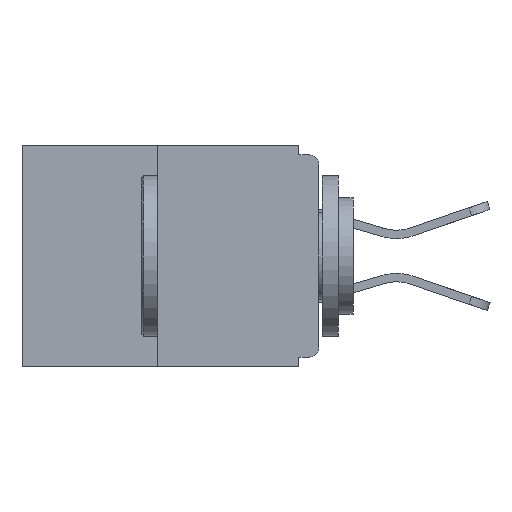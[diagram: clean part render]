
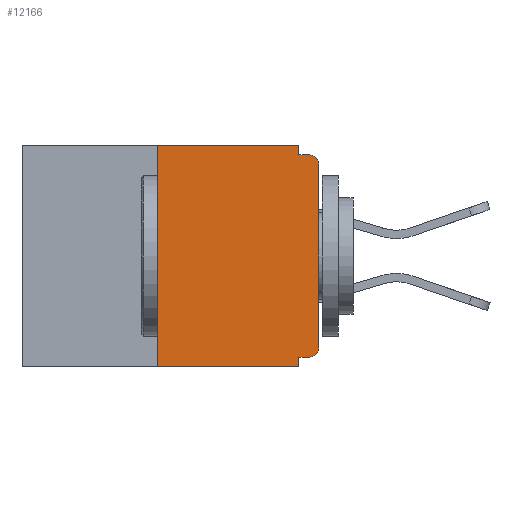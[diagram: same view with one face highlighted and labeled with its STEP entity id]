
A CAD part, left-side view. The second image highlights one B-rep face of the part: STEP entity #12166.
In plain terms, the highlighted planar face has unit normal (-1, 0, 0).
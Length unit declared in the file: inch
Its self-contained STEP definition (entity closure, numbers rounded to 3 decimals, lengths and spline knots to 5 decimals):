
#251 = EDGE_CURVE ( 'NONE', #6789, #2099, #13063, .T. ) ;
#456 = VERTEX_POINT ( 'NONE', #16855 ) ;
#589 = CARTESIAN_POINT ( 'NONE',  ( 0., 0.031, -0.015 ) ) ;
#648 = VECTOR ( 'NONE', #12299, 39.37008 ) ;
#949 = CARTESIAN_POINT ( 'NONE',  ( 0., 0.46, -0.343 ) ) ;
#1015 = DIRECTION ( 'NONE',  ( 0., -1., 0. ) ) ;
#1018 = ORIENTED_EDGE ( 'NONE', *, *, #12444, .F. ) ;
#1489 = ORIENTED_EDGE ( 'NONE', *, *, #14130, .F. ) ;
#1553 = ORIENTED_EDGE ( 'NONE', *, *, #16051, .T. ) ;
#2029 = VECTOR ( 'NONE', #5635, 39.37008 ) ;
#2099 = VERTEX_POINT ( 'NONE', #11036 ) ;
#2513 = CARTESIAN_POINT ( 'NONE',  ( 0., 0.031, -0.328 ) ) ;
#2523 = VECTOR ( 'NONE', #14605, 39.37008 ) ;
#3146 = VERTEX_POINT ( 'NONE', #15047 ) ;
#3176 = VECTOR ( 'NONE', #1015, 39.37008 ) ;
#3281 = EDGE_LOOP ( 'NONE', ( #15553, #9394, #1553, #1018, #1489, #11393, #9842, #7065, #14509, #13046 ) ) ;
#4202 = CARTESIAN_POINT ( 'NONE',  ( 0., 0.031, 0. ) ) ;
#5271 = CARTESIAN_POINT ( 'NONE',  ( 0., 0.031, 0. ) ) ;
#5534 = CARTESIAN_POINT ( 'NONE',  ( 0., 0.25, -0.343 ) ) ;
#5581 = DIRECTION ( 'NONE',  ( 0., -1., 0. ) ) ;
#5635 = DIRECTION ( 'NONE',  ( 0., 0., -1. ) ) ;
#5746 = VECTOR ( 'NONE', #5581, 39.37008 ) ;
#5886 = LINE ( 'NONE', #949, #3176 ) ;
#6510 = AXIS2_PLACEMENT_3D ( 'NONE', #8123, #16675, #8061 ) ;
#6789 = VERTEX_POINT ( 'NONE', #589 ) ;
#6872 = AXIS2_PLACEMENT_3D ( 'NONE', #17075, #10003, #14261 ) ;
#7065 = ORIENTED_EDGE ( 'NONE', *, *, #11221, .T. ) ;
#7157 = LINE ( 'NONE', #15218, #18271 ) ;
#7294 = CIRCLE ( 'NONE', #6872, 0.015 ) ;
#7665 = VERTEX_POINT ( 'NONE', #11870 ) ;
#7759 = EDGE_CURVE ( 'NONE', #15912, #6789, #17613, .T. ) ;
#8061 = DIRECTION ( 'NONE',  ( 0., 0., -1. ) ) ;
#8123 = CARTESIAN_POINT ( 'NONE',  ( 0., 0.46, 0. ) ) ;
#8216 = EDGE_CURVE ( 'NONE', #7665, #18246, #7157, .T. ) ;
#9111 = CIRCLE ( 'NONE', #14252, 0.015 ) ;
#9394 = ORIENTED_EDGE ( 'NONE', *, *, #18094, .F. ) ;
#9842 = ORIENTED_EDGE ( 'NONE', *, *, #8216, .T. ) ;
#10003 = DIRECTION ( 'NONE',  ( -1., 0., 0. ) ) ;
#10218 = VECTOR ( 'NONE', #15487, 39.37008 ) ;
#10864 = CARTESIAN_POINT ( 'NONE',  ( 0., 0., -0.03 ) ) ;
#11036 = CARTESIAN_POINT ( 'NONE',  ( 0., 0.015, -0.015 ) ) ;
#11221 = EDGE_CURVE ( 'NONE', #18246, #2099, #7294, .T. ) ;
#11393 = ORIENTED_EDGE ( 'NONE', *, *, #17899, .T. ) ;
#11527 = LINE ( 'NONE', #12703, #5746 ) ;
#11870 = CARTESIAN_POINT ( 'NONE',  ( 0., 0., -0.313 ) ) ;
#12135 = FACE_OUTER_BOUND ( 'NONE', #3281, .T. ) ;
#12145 = VECTOR ( 'NONE', #15330, 39.37008 ) ;
#12166 = ADVANCED_FACE ( 'NONE', ( #12135 ), #16099, .F. ) ;
#12299 = DIRECTION ( 'NONE',  ( 0., 1., 0. ) ) ;
#12444 = EDGE_CURVE ( 'NONE', #13809, #456, #14600, .T. ) ;
#12703 = CARTESIAN_POINT ( 'NONE',  ( 0., 0.46, 0. ) ) ;
#12765 = VERTEX_POINT ( 'NONE', #5534 ) ;
#13046 = ORIENTED_EDGE ( 'NONE', *, *, #7759, .F. ) ;
#13063 = LINE ( 'NONE', #18193, #12145 ) ;
#13226 = CARTESIAN_POINT ( 'NONE',  ( 0., 0.015, -0.313 ) ) ;
#13809 = VERTEX_POINT ( 'NONE', #2513 ) ;
#13900 = EDGE_CURVE ( 'NONE', #14069, #15912, #11527, .T. ) ;
#14011 = CARTESIAN_POINT ( 'NONE',  ( 0., 0.25, 0. ) ) ;
#14069 = VERTEX_POINT ( 'NONE', #17996 ) ;
#14130 = EDGE_CURVE ( 'NONE', #3146, #13809, #14848, .T. ) ;
#14252 = AXIS2_PLACEMENT_3D ( 'NONE', #13226, #14586, #14643 ) ;
#14261 = DIRECTION ( 'NONE',  ( 0., 0., -1. ) ) ;
#14509 = ORIENTED_EDGE ( 'NONE', *, *, #251, .F. ) ;
#14586 = DIRECTION ( 'NONE',  ( -1., 0., 0. ) ) ;
#14600 = LINE ( 'NONE', #17318, #2523 ) ;
#14605 = DIRECTION ( 'NONE',  ( 0., 0., -1. ) ) ;
#14643 = DIRECTION ( 'NONE',  ( 0., 0., -1. ) ) ;
#14848 = LINE ( 'NONE', #15141, #648 ) ;
#15047 = CARTESIAN_POINT ( 'NONE',  ( 0., 0.015, -0.328 ) ) ;
#15141 = CARTESIAN_POINT ( 'NONE',  ( 0., 0., -0.328 ) ) ;
#15218 = CARTESIAN_POINT ( 'NONE',  ( 0., 0., 0. ) ) ;
#15330 = DIRECTION ( 'NONE',  ( 0., -1., 0. ) ) ;
#15487 = DIRECTION ( 'NONE',  ( 0., 0., 1. ) ) ;
#15553 = ORIENTED_EDGE ( 'NONE', *, *, #13900, .F. ) ;
#15912 = VERTEX_POINT ( 'NONE', #5271 ) ;
#16051 = EDGE_CURVE ( 'NONE', #12765, #456, #5886, .T. ) ;
#16099 = PLANE ( 'NONE',  #6510 ) ;
#16675 = DIRECTION ( 'NONE',  ( 1., 0., 0. ) ) ;
#16855 = CARTESIAN_POINT ( 'NONE',  ( 0., 0.031, -0.343 ) ) ;
#17075 = CARTESIAN_POINT ( 'NONE',  ( 0., 0.015, -0.03 ) ) ;
#17318 = CARTESIAN_POINT ( 'NONE',  ( 0., 0.031, -0.343 ) ) ;
#17579 = LINE ( 'NONE', #14011, #10218 ) ;
#17613 = LINE ( 'NONE', #4202, #2029 ) ;
#17899 = EDGE_CURVE ( 'NONE', #3146, #7665, #9111, .T. ) ;
#17996 = CARTESIAN_POINT ( 'NONE',  ( 0., 0.25, 0. ) ) ;
#18094 = EDGE_CURVE ( 'NONE', #12765, #14069, #17579, .T. ) ;
#18193 = CARTESIAN_POINT ( 'NONE',  ( 0., 0., -0.015 ) ) ;
#18206 = DIRECTION ( 'NONE',  ( 0., 0., 1. ) ) ;
#18246 = VERTEX_POINT ( 'NONE', #10864 ) ;
#18271 = VECTOR ( 'NONE', #18206, 39.37008 ) ;
